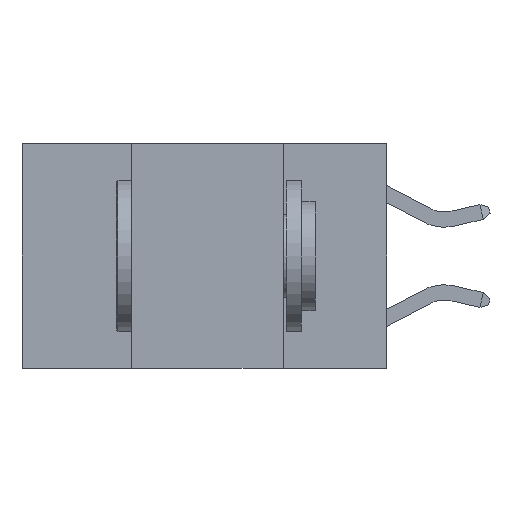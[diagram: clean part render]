
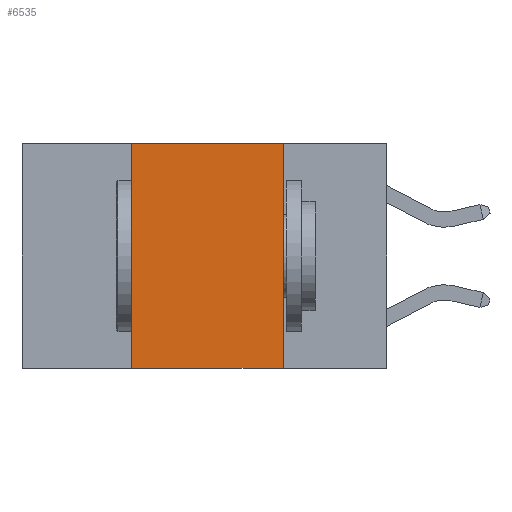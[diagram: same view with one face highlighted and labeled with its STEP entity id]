
A CAD part, left-side view. The second image highlights one B-rep face of the part: STEP entity #6535.
In plain terms, the highlighted planar face has unit normal (-1, 0, 0).
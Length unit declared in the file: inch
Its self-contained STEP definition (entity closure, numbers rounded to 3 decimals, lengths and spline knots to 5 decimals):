
#100 = VERTEX_POINT ( 'NONE', #7257 ) ;
#749 = DIRECTION ( 'NONE',  ( 0., 0., 1. ) ) ;
#888 = VECTOR ( 'NONE', #6448, 39.37008 ) ;
#1746 = LINE ( 'NONE', #15577, #888 ) ;
#1848 = DIRECTION ( 'NONE',  ( 1., 0., 0. ) ) ;
#2018 = VERTEX_POINT ( 'NONE', #14206 ) ;
#2071 = EDGE_CURVE ( 'NONE', #2018, #100, #1746, .T. ) ;
#2734 = VECTOR ( 'NONE', #3015, 39.37008 ) ;
#3015 = DIRECTION ( 'NONE',  ( 0., -1., 0. ) ) ;
#3512 = ORIENTED_EDGE ( 'NONE', *, *, #13868, .T. ) ;
#4465 = PLANE ( 'NONE',  #7379 ) ;
#5063 = VERTEX_POINT ( 'NONE', #11885 ) ;
#5624 = LINE ( 'NONE', #15203, #12143 ) ;
#5916 = VECTOR ( 'NONE', #749, 39.37008 ) ;
#6448 = DIRECTION ( 'NONE',  ( 0., 0., -1. ) ) ;
#6471 = EDGE_CURVE ( 'NONE', #5063, #2018, #16277, .T. ) ;
#6535 = ADVANCED_FACE ( 'NONE', ( #11972 ), #4465, .F. ) ;
#7257 = CARTESIAN_POINT ( 'NONE',  ( 0., 0.17, -0.37 ) ) ;
#7366 = CARTESIAN_POINT ( 'NONE',  ( 0., 0.42, 0. ) ) ;
#7379 = AXIS2_PLACEMENT_3D ( 'NONE', #14944, #1848, #11032 ) ;
#8328 = CARTESIAN_POINT ( 'NONE',  ( 0., 0.6, 0. ) ) ;
#8683 = DIRECTION ( 'NONE',  ( 0., -1., 0. ) ) ;
#9097 = VERTEX_POINT ( 'NONE', #13003 ) ;
#9653 = ORIENTED_EDGE ( 'NONE', *, *, #10991, .F. ) ;
#10645 = EDGE_LOOP ( 'NONE', ( #11487, #11913, #9653, #3512 ) ) ;
#10991 = EDGE_CURVE ( 'NONE', #9097, #5063, #13684, .T. ) ;
#11032 = DIRECTION ( 'NONE',  ( 0., 0., -1. ) ) ;
#11487 = ORIENTED_EDGE ( 'NONE', *, *, #2071, .F. ) ;
#11885 = CARTESIAN_POINT ( 'NONE',  ( 0., 0.42, 0. ) ) ;
#11913 = ORIENTED_EDGE ( 'NONE', *, *, #6471, .F. ) ;
#11972 = FACE_OUTER_BOUND ( 'NONE', #10645, .T. ) ;
#12143 = VECTOR ( 'NONE', #8683, 39.37008 ) ;
#13003 = CARTESIAN_POINT ( 'NONE',  ( 0., 0.42, -0.37 ) ) ;
#13684 = LINE ( 'NONE', #7366, #5916 ) ;
#13868 = EDGE_CURVE ( 'NONE', #9097, #100, #5624, .T. ) ;
#14206 = CARTESIAN_POINT ( 'NONE',  ( 0., 0.17, 0. ) ) ;
#14944 = CARTESIAN_POINT ( 'NONE',  ( 0., 0.6, 0. ) ) ;
#15203 = CARTESIAN_POINT ( 'NONE',  ( 0., 0.6, -0.37 ) ) ;
#15577 = CARTESIAN_POINT ( 'NONE',  ( 0., 0.17, 0. ) ) ;
#16277 = LINE ( 'NONE', #8328, #2734 ) ;
